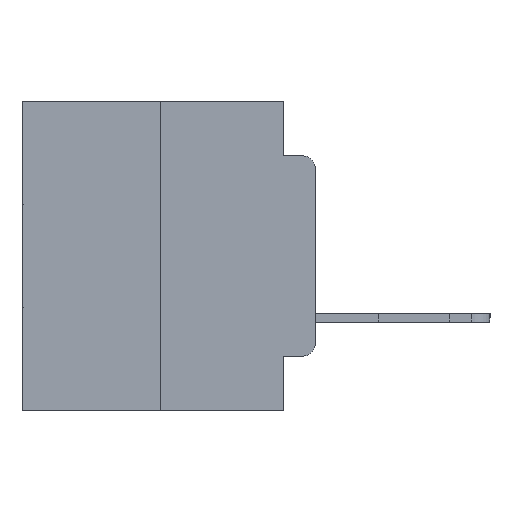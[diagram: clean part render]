
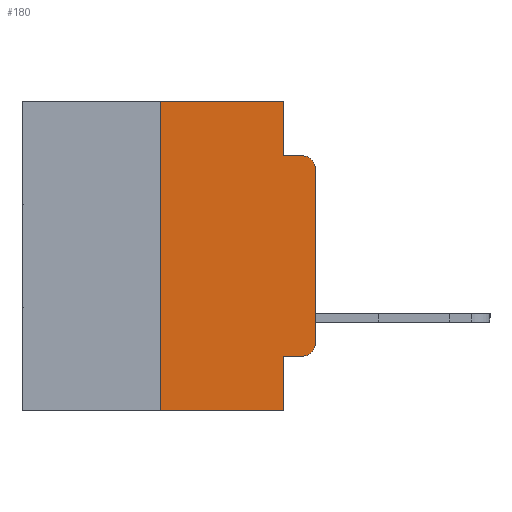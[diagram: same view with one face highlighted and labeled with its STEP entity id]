
A CAD part, left-side view. The second image highlights one B-rep face of the part: STEP entity #180.
In plain terms, the highlighted planar face has unit normal (-1, 0, 0).
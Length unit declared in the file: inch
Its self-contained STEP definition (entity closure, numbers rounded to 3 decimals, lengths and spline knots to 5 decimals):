
#180 = ADVANCED_FACE ( 'NONE', ( #11631 ), #23293, .F. ) ;
#830 = CARTESIAN_POINT ( 'NONE',  ( 0., 0.25, 0. ) ) ;
#1151 = DIRECTION ( 'NONE',  ( 0., 0., -1. ) ) ;
#1238 = LINE ( 'NONE', #5981, #18727 ) ;
#1650 = CARTESIAN_POINT ( 'NONE',  ( 0., 0.02, -0.4115 ) ) ;
#1660 = DIRECTION ( 'NONE',  ( 0., 0., 1. ) ) ;
#1754 = VERTEX_POINT ( 'NONE', #17387 ) ;
#2560 = LINE ( 'NONE', #830, #14256 ) ;
#2875 = VECTOR ( 'NONE', #10778, 39.37008 ) ;
#3079 = VERTEX_POINT ( 'NONE', #20860 ) ;
#3429 = EDGE_CURVE ( 'NONE', #4039, #3079, #16917, .T. ) ;
#4039 = VERTEX_POINT ( 'NONE', #12243 ) ;
#4331 = VERTEX_POINT ( 'NONE', #26464 ) ;
#4371 = CARTESIAN_POINT ( 'NONE',  ( 0., 0.02, -0.3915 ) ) ;
#4433 = VERTEX_POINT ( 'NONE', #24594 ) ;
#5343 = VECTOR ( 'NONE', #1660, 39.37008 ) ;
#5673 = ORIENTED_EDGE ( 'NONE', *, *, #19951, .T. ) ;
#5846 = CARTESIAN_POINT ( 'NONE',  ( 0., 0.25, 0. ) ) ;
#5912 = CIRCLE ( 'NONE', #8233, 0.02 ) ;
#5981 = CARTESIAN_POINT ( 'NONE',  ( 0., 0.051, 0. ) ) ;
#6170 = CARTESIAN_POINT ( 'NONE',  ( 0., 0., -0.1085 ) ) ;
#6176 = VERTEX_POINT ( 'NONE', #5846 ) ;
#6247 = CARTESIAN_POINT ( 'NONE',  ( 0., 0.473, 0. ) ) ;
#6564 = DIRECTION ( 'NONE',  ( 0., 0., -1. ) ) ;
#8011 = ORIENTED_EDGE ( 'NONE', *, *, #28188, .F. ) ;
#8057 = CARTESIAN_POINT ( 'NONE',  ( 0., 0.02, -0.1085 ) ) ;
#8182 = CARTESIAN_POINT ( 'NONE',  ( 0., 0.25, -0.5 ) ) ;
#8233 = AXIS2_PLACEMENT_3D ( 'NONE', #8057, #23419, #10263 ) ;
#8245 = DIRECTION ( 'NONE',  ( 0., -1., 0. ) ) ;
#8440 = ORIENTED_EDGE ( 'NONE', *, *, #3429, .F. ) ;
#8681 = LINE ( 'NONE', #10689, #2875 ) ;
#8895 = LINE ( 'NONE', #9280, #26383 ) ;
#9280 = CARTESIAN_POINT ( 'NONE',  ( 0., 0.051, -0.4115 ) ) ;
#9646 = EDGE_CURVE ( 'NONE', #28178, #1754, #10872, .T. ) ;
#10263 = DIRECTION ( 'NONE',  ( 0., 0., -1. ) ) ;
#10368 = VECTOR ( 'NONE', #1151, 39.37008 ) ;
#10673 = ORIENTED_EDGE ( 'NONE', *, *, #20367, .T. ) ;
#10689 = CARTESIAN_POINT ( 'NONE',  ( 0., 0.051, -0.0885 ) ) ;
#10778 = DIRECTION ( 'NONE',  ( 0., -1., 0. ) ) ;
#10872 = LINE ( 'NONE', #21418, #17431 ) ;
#10922 = EDGE_CURVE ( 'NONE', #15958, #1754, #1238, .T. ) ;
#10956 = LINE ( 'NONE', #12615, #16819 ) ;
#11631 = FACE_OUTER_BOUND ( 'NONE', #19710, .T. ) ;
#12243 = CARTESIAN_POINT ( 'NONE',  ( 0., 0.051, 0. ) ) ;
#12615 = CARTESIAN_POINT ( 'NONE',  ( 0., 0.473, 0. ) ) ;
#12628 = EDGE_CURVE ( 'NONE', #3079, #4433, #8681, .T. ) ;
#13982 = DIRECTION ( 'NONE',  ( 0., 0., 1. ) ) ;
#14256 = VECTOR ( 'NONE', #13982, 39.37008 ) ;
#14850 = DIRECTION ( 'NONE',  ( 0., -1., 0. ) ) ;
#15958 = VERTEX_POINT ( 'NONE', #22039 ) ;
#16281 = ORIENTED_EDGE ( 'NONE', *, *, #25077, .F. ) ;
#16446 = VERTEX_POINT ( 'NONE', #6170 ) ;
#16819 = VECTOR ( 'NONE', #14850, 39.37008 ) ;
#16917 = LINE ( 'NONE', #17928, #10368 ) ;
#16974 = CARTESIAN_POINT ( 'NONE',  ( 0., 0., 0. ) ) ;
#17031 = ORIENTED_EDGE ( 'NONE', *, *, #12628, .F. ) ;
#17387 = CARTESIAN_POINT ( 'NONE',  ( 0., 0.051, -0.5 ) ) ;
#17431 = VECTOR ( 'NONE', #8245, 39.37008 ) ;
#17928 = CARTESIAN_POINT ( 'NONE',  ( 0., 0.051, 0. ) ) ;
#18193 = AXIS2_PLACEMENT_3D ( 'NONE', #4371, #19721, #6564 ) ;
#18315 = ORIENTED_EDGE ( 'NONE', *, *, #24093, .T. ) ;
#18405 = LINE ( 'NONE', #16974, #5343 ) ;
#18727 = VECTOR ( 'NONE', #27877, 39.37008 ) ;
#18732 = ORIENTED_EDGE ( 'NONE', *, *, #21796, .T. ) ;
#19710 = EDGE_LOOP ( 'NONE', ( #18315, #10673, #17031, #8440, #8011, #16281, #25827, #24858, #18732, #5673 ) ) ;
#19721 = DIRECTION ( 'NONE',  ( -1., 0., 0. ) ) ;
#19951 = EDGE_CURVE ( 'NONE', #25983, #4331, #24120, .T. ) ;
#20367 = EDGE_CURVE ( 'NONE', #16446, #4433, #5912, .T. ) ;
#20757 = DIRECTION ( 'NONE',  ( 0., 0., -1. ) ) ;
#20860 = CARTESIAN_POINT ( 'NONE',  ( 0., 0.051, -0.0885 ) ) ;
#21418 = CARTESIAN_POINT ( 'NONE',  ( 0., 0.473, -0.5 ) ) ;
#21796 = EDGE_CURVE ( 'NONE', #15958, #25983, #8895, .T. ) ;
#22039 = CARTESIAN_POINT ( 'NONE',  ( 0., 0.051, -0.4115 ) ) ;
#22072 = AXIS2_PLACEMENT_3D ( 'NONE', #6247, #22200, #20757 ) ;
#22200 = DIRECTION ( 'NONE',  ( 1., 0., 0. ) ) ;
#22451 = DIRECTION ( 'NONE',  ( 0., -1., 0. ) ) ;
#23293 = PLANE ( 'NONE',  #22072 ) ;
#23419 = DIRECTION ( 'NONE',  ( -1., 0., 0. ) ) ;
#24093 = EDGE_CURVE ( 'NONE', #4331, #16446, #18405, .T. ) ;
#24120 = CIRCLE ( 'NONE', #18193, 0.02 ) ;
#24594 = CARTESIAN_POINT ( 'NONE',  ( 0., 0.02, -0.0885 ) ) ;
#24858 = ORIENTED_EDGE ( 'NONE', *, *, #10922, .F. ) ;
#25077 = EDGE_CURVE ( 'NONE', #28178, #6176, #2560, .T. ) ;
#25827 = ORIENTED_EDGE ( 'NONE', *, *, #9646, .T. ) ;
#25983 = VERTEX_POINT ( 'NONE', #1650 ) ;
#26383 = VECTOR ( 'NONE', #22451, 39.37008 ) ;
#26464 = CARTESIAN_POINT ( 'NONE',  ( 0., 0., -0.3915 ) ) ;
#27877 = DIRECTION ( 'NONE',  ( 0., 0., -1. ) ) ;
#28178 = VERTEX_POINT ( 'NONE', #8182 ) ;
#28188 = EDGE_CURVE ( 'NONE', #6176, #4039, #10956, .T. ) ;
